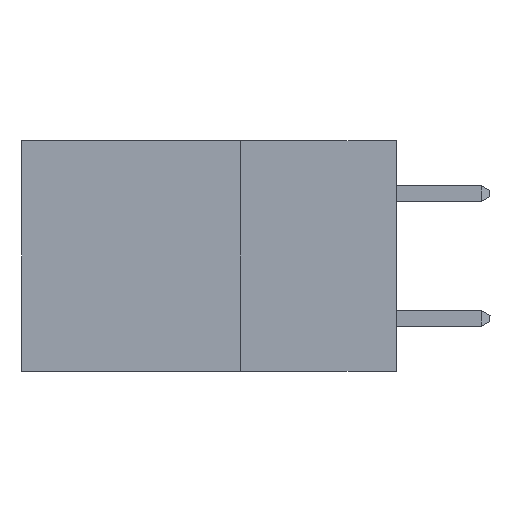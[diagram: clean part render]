
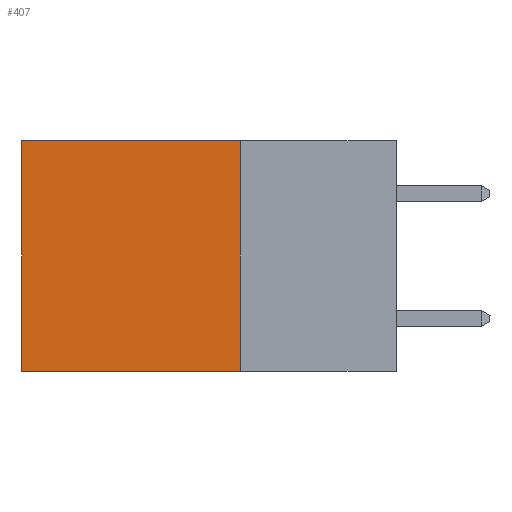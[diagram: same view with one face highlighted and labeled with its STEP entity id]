
A CAD part, left-side view. The second image highlights one B-rep face of the part: STEP entity #407.
In plain terms, the highlighted planar face has unit normal (-1, 0, 0).
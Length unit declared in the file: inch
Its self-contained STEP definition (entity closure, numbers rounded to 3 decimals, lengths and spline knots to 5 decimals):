
#407 = ADVANCED_FACE ( 'NONE', ( #14336 ), #9532, .F. ) ;
#456 = VERTEX_POINT ( 'NONE', #11304 ) ;
#568 = CARTESIAN_POINT ( 'NONE',  ( 0.298, 0.25, -0.37 ) ) ;
#1312 = VERTEX_POINT ( 'NONE', #568 ) ;
#1433 = ORIENTED_EDGE ( 'NONE', *, *, #12780, .F. ) ;
#2397 = ORIENTED_EDGE ( 'NONE', *, *, #11521, .T. ) ;
#3413 = VERTEX_POINT ( 'NONE', #20032 ) ;
#3488 = DIRECTION ( 'NONE',  ( 0., 0., -1. ) ) ;
#3617 = VECTOR ( 'NONE', #11256, 39.37008 ) ;
#4209 = CARTESIAN_POINT ( 'NONE',  ( 0.298, 0.6, 0. ) ) ;
#4749 = LINE ( 'NONE', #18603, #19170 ) ;
#5445 = VECTOR ( 'NONE', #3488, 39.37008 ) ;
#7264 = CARTESIAN_POINT ( 'NONE',  ( 0.298, 0.25, 0. ) ) ;
#7558 = DIRECTION ( 'NONE',  ( 0., 0., -1. ) ) ;
#8513 = VECTOR ( 'NONE', #7558, 39.37008 ) ;
#8609 = EDGE_LOOP ( 'NONE', ( #18722, #16039, #1433, #2397 ) ) ;
#9532 = PLANE ( 'NONE',  #12015 ) ;
#9855 = CARTESIAN_POINT ( 'NONE',  ( 0.298, 0.6, 0. ) ) ;
#11170 = CARTESIAN_POINT ( 'NONE',  ( 0.298, 0.25, 0. ) ) ;
#11256 = DIRECTION ( 'NONE',  ( 0., 1., 0. ) ) ;
#11304 = CARTESIAN_POINT ( 'NONE',  ( 0.298, 0.6, -0.37 ) ) ;
#11521 = EDGE_CURVE ( 'NONE', #3413, #12092, #4749, .T. ) ;
#12015 = AXIS2_PLACEMENT_3D ( 'NONE', #11170, #20676, #14329 ) ;
#12092 = VERTEX_POINT ( 'NONE', #4209 ) ;
#12780 = EDGE_CURVE ( 'NONE', #3413, #1312, #12855, .T. ) ;
#12855 = LINE ( 'NONE', #7264, #8513 ) ;
#13980 = LINE ( 'NONE', #16244, #3617 ) ;
#14329 = DIRECTION ( 'NONE',  ( 0., 0., -1. ) ) ;
#14336 = FACE_OUTER_BOUND ( 'NONE', #8609, .T. ) ;
#16039 = ORIENTED_EDGE ( 'NONE', *, *, #18830, .F. ) ;
#16244 = CARTESIAN_POINT ( 'NONE',  ( 0.298, 0.25, -0.37 ) ) ;
#18315 = LINE ( 'NONE', #9855, #5445 ) ;
#18539 = DIRECTION ( 'NONE',  ( 0., 1., 0. ) ) ;
#18603 = CARTESIAN_POINT ( 'NONE',  ( 0.298, 0.25, 0. ) ) ;
#18722 = ORIENTED_EDGE ( 'NONE', *, *, #20747, .T. ) ;
#18830 = EDGE_CURVE ( 'NONE', #1312, #456, #13980, .T. ) ;
#19170 = VECTOR ( 'NONE', #18539, 39.37008 ) ;
#20032 = CARTESIAN_POINT ( 'NONE',  ( 0.298, 0.25, 0. ) ) ;
#20676 = DIRECTION ( 'NONE',  ( 1., 0., 0. ) ) ;
#20747 = EDGE_CURVE ( 'NONE', #12092, #456, #18315, .T. ) ;
